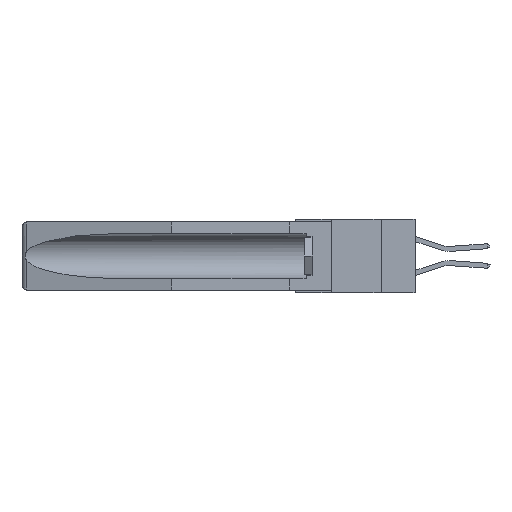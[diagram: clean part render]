
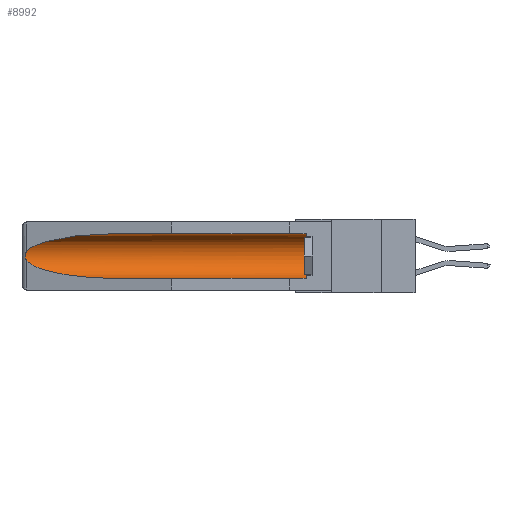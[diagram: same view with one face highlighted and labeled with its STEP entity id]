
A CAD part, left-side view. The second image highlights one B-rep face of the part: STEP entity #8992.
In plain terms, the highlighted cylindrical face has radius 2.857 mm (diameter 5.715 mm), a partial arc.
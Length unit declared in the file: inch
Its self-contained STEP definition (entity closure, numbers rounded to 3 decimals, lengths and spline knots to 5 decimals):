
#74 = CARTESIAN_POINT ( 'NONE',  ( 0.155, -0.30754, -0.1715 ) ) ;
#584 = VECTOR ( 'NONE', #7601, 39.37008 ) ;
#1026 = ORIENTED_EDGE ( 'NONE', *, *, #8932, .F. ) ;
#2311 = ORIENTED_EDGE ( 'NONE', *, *, #15842, .T. ) ;
#2578 = VERTEX_POINT ( 'NONE', #14618 ) ;
#3037 = CARTESIAN_POINT ( 'NONE',  ( 0.2673, 1.53269, -0.17917 ) ) ;
#3200 = CARTESIAN_POINT ( 'NONE',  ( 0.155, 0.126, -0.1715 ) ) ;
#3329 = DIRECTION ( 'NONE',  ( 0., 0., 1. ) ) ;
#3508 = AXIS2_PLACEMENT_3D ( 'NONE', #74, #11453, #3329 ) ;
#3595 = EDGE_CURVE ( 'NONE', #2578, #7830, #19050, .T. ) ;
#4107 = CARTESIAN_POINT ( 'NONE',  ( 0.21114, 1.30732, -0.284 ) ) ;
#4505 = CARTESIAN_POINT ( 'NONE',  ( 0.21114, 1.30732, -0.059 ) ) ;
#4584 = CARTESIAN_POINT ( 'NONE',  ( 0.25451, 1.48313, -0.09465 ) ) ;
#4739 = CYLINDRICAL_SURFACE ( 'NONE', #3508, 0.1125 ) ;
#4970 = CARTESIAN_POINT ( 'NONE',  ( 0.26537, 1.52718, -0.14972 ) ) ;
#5049 = CARTESIAN_POINT ( 'NONE',  ( 0.155, 1.07973, -0.059 ) ) ;
#5360 = CARTESIAN_POINT ( 'NONE',  ( 0.155, -0.30754, -0.059 ) ) ;
#7067 = ORIENTED_EDGE ( 'NONE', *, *, #17442, .T. ) ;
#7097 = VERTEX_POINT ( 'NONE', #4970 ) ;
#7391 = EDGE_CURVE ( 'NONE', #19943, #7097, #14285, .T. ) ;
#7561 = CARTESIAN_POINT ( 'NONE',  ( 0.155, 1.07973, -0.059 ) ) ;
#7601 = DIRECTION ( 'NONE',  ( 0., 1., 0. ) ) ;
#7642 = LINE ( 'NONE', #5360, #16483 ) ;
#7699 = ORIENTED_EDGE ( 'NONE', *, *, #7391, .T. ) ;
#7830 = VERTEX_POINT ( 'NONE', #15861 ) ;
#7854 = CARTESIAN_POINT ( 'NONE',  ( 0.26537, 1.52718, -0.14972 ) ) ;
#8102 = CARTESIAN_POINT ( 'NONE',  ( 0.26597, 1.5296, -0.19026 ) ) ;
#8877 = AXIS2_PLACEMENT_3D ( 'NONE', #3200, #16009, #9587 ) ;
#8932 = EDGE_CURVE ( 'NONE', #2578, #20542, #15832, .T. ) ;
#8992 = ADVANCED_FACE ( 'NONE', ( #20126 ), #4739, .F. ) ;
#9110 = B_SPLINE_CURVE_WITH_KNOTS ( 'NONE', 3,
 ( #10958, #17321, #11104, #17740, #14355, #12654, #3037, #11311, #8102, #19375 ),
 .UNSPECIFIED., .F., .F.,
 ( 4, 2, 2, 2, 4 ),
 ( 0., 0.00029, 0.00058, 0.00087, 0.00117 ),
 .UNSPECIFIED. ) ;
#9587 = DIRECTION ( 'NONE',  ( 0., 0., 1. ) ) ;
#9835 = EDGE_CURVE ( 'NONE', #7097, #16770, #9110, .T. ) ;
#10958 = CARTESIAN_POINT ( 'NONE',  ( 0.26537, 1.52718, -0.14972 ) ) ;
#11104 = CARTESIAN_POINT ( 'NONE',  ( 0.26654, 1.53092, -0.15636 ) ) ;
#11311 = CARTESIAN_POINT ( 'NONE',  ( 0.26655, 1.53094, -0.18657 ) ) ;
#11448 = CARTESIAN_POINT ( 'NONE',  ( 0.26537, 1.52718, -0.19328 ) ) ;
#11453 = DIRECTION ( 'NONE',  ( 0., 1., 0. ) ) ;
#12654 = CARTESIAN_POINT ( 'NONE',  ( 0.2675, 1.53308, -0.17534 ) ) ;
#13097 = CARTESIAN_POINT ( 'NONE',  ( 0.155, 1.07973, -0.284 ) ) ;
#13367 = EDGE_LOOP ( 'NONE', ( #7699, #20730, #7067, #1026, #18764, #2311 ) ) ;
#13864 = CARTESIAN_POINT ( 'NONE',  ( 0.26537, 1.52718, -0.19328 ) ) ;
#14138 =( BOUNDED_CURVE ( )  B_SPLINE_CURVE ( 3, ( #13864, #17250, #4107, #17110 ),
 .UNSPECIFIED., .F., .F. ) 
 B_SPLINE_CURVE_WITH_KNOTS ( ( 4, 4 ),
 ( 0.1948, 1.5708 ),
 .UNSPECIFIED. ) 
 CURVE ( )  GEOMETRIC_REPRESENTATION_ITEM ( )  RATIONAL_B_SPLINE_CURVE ( ( 1., 0.848, 0.848, 1. ) ) 
 REPRESENTATION_ITEM ( '' )  );
#14285 =( BOUNDED_CURVE ( )  B_SPLINE_CURVE ( 3, ( #7561, #4505, #4584, #7854 ),
 .UNSPECIFIED., .F., .F. ) 
 B_SPLINE_CURVE_WITH_KNOTS ( ( 4, 4 ),
 ( 4.71239, 6.08839 ),
 .UNSPECIFIED. ) 
 CURVE ( )  GEOMETRIC_REPRESENTATION_ITEM ( )  RATIONAL_B_SPLINE_CURVE ( ( 1., 0.848, 0.848, 1. ) ) 
 REPRESENTATION_ITEM ( '' )  );
#14355 = CARTESIAN_POINT ( 'NONE',  ( 0.2675, 1.53308, -0.16763 ) ) ;
#14618 = CARTESIAN_POINT ( 'NONE',  ( 0.155, 0.126, -0.284 ) ) ;
#15644 = CARTESIAN_POINT ( 'NONE',  ( 0.155, -0.30754, -0.284 ) ) ;
#15832 = LINE ( 'NONE', #15644, #584 ) ;
#15842 = EDGE_CURVE ( 'NONE', #7830, #19943, #7642, .T. ) ;
#15861 = CARTESIAN_POINT ( 'NONE',  ( 0.155, 0.126, -0.059 ) ) ;
#16009 = DIRECTION ( 'NONE',  ( 0., -1., 0. ) ) ;
#16380 = DIRECTION ( 'NONE',  ( 0., 1., 0. ) ) ;
#16483 = VECTOR ( 'NONE', #16380, 39.37008 ) ;
#16770 = VERTEX_POINT ( 'NONE', #11448 ) ;
#17110 = CARTESIAN_POINT ( 'NONE',  ( 0.155, 1.07973, -0.284 ) ) ;
#17250 = CARTESIAN_POINT ( 'NONE',  ( 0.25451, 1.48313, -0.24835 ) ) ;
#17321 = CARTESIAN_POINT ( 'NONE',  ( 0.26597, 1.52961, -0.15275 ) ) ;
#17442 = EDGE_CURVE ( 'NONE', #16770, #20542, #14138, .T. ) ;
#17740 = CARTESIAN_POINT ( 'NONE',  ( 0.2673, 1.5327, -0.16383 ) ) ;
#18764 = ORIENTED_EDGE ( 'NONE', *, *, #3595, .T. ) ;
#19050 = CIRCLE ( 'NONE', #8877, 0.1125 ) ;
#19375 = CARTESIAN_POINT ( 'NONE',  ( 0.26537, 1.52718, -0.19328 ) ) ;
#19943 = VERTEX_POINT ( 'NONE', #5049 ) ;
#20126 = FACE_OUTER_BOUND ( 'NONE', #13367, .T. ) ;
#20542 = VERTEX_POINT ( 'NONE', #13097 ) ;
#20730 = ORIENTED_EDGE ( 'NONE', *, *, #9835, .T. ) ;
